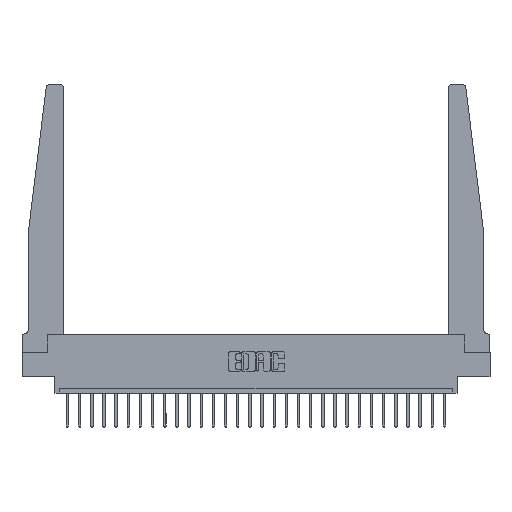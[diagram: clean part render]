
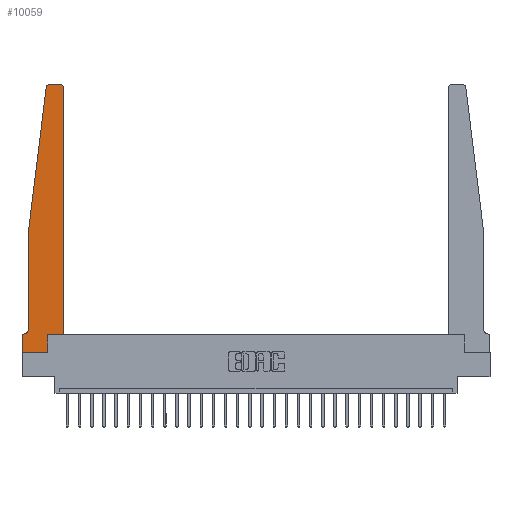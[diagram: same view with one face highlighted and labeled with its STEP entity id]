
A CAD part, top view. The second image highlights one B-rep face of the part: STEP entity #10059.
In plain terms, the highlighted planar face has unit normal (0, 0, 1).
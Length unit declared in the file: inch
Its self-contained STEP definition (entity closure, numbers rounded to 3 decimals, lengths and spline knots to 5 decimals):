
#682 = LINE ( 'NONE', #19217, #24742 ) ;
#1651 = DIRECTION ( 'NONE',  ( 0., 0., 1. ) ) ;
#1789 = DIRECTION ( 'NONE',  ( 1., 0., 0. ) ) ;
#1814 = LINE ( 'NONE', #2069, #9241 ) ;
#2069 = CARTESIAN_POINT ( 'NONE',  ( 0.065, 1.25, 0.37 ) ) ;
#2186 = ORIENTED_EDGE ( 'NONE', *, *, #5775, .T. ) ;
#2932 = VERTEX_POINT ( 'NONE', #6371 ) ;
#2943 = ORIENTED_EDGE ( 'NONE', *, *, #3992, .T. ) ;
#3528 = ORIENTED_EDGE ( 'NONE', *, *, #22419, .T. ) ;
#3712 = DIRECTION ( 'NONE',  ( 0., 0., 1. ) ) ;
#3728 = LINE ( 'NONE', #24303, #25688 ) ;
#3889 = DIRECTION ( 'NONE',  ( 0., 0., 1. ) ) ;
#3896 = CARTESIAN_POINT ( 'NONE',  ( 0., 0.1875, 0.37 ) ) ;
#3992 = EDGE_CURVE ( 'NONE', #25534, #2932, #1814, .T. ) ;
#4016 = ORIENTED_EDGE ( 'NONE', *, *, #21469, .T. ) ;
#4649 = CARTESIAN_POINT ( 'NONE',  ( 0.24675, 2.72367, 0.37 ) ) ;
#4956 = LINE ( 'NONE', #25655, #26504 ) ;
#5046 = AXIS2_PLACEMENT_3D ( 'NONE', #5643, #3889, #5364 ) ;
#5364 = DIRECTION ( 'NONE',  ( 1., 0., 0. ) ) ;
#5643 = CARTESIAN_POINT ( 'NONE',  ( 0.27653, 2.72, 0.37 ) ) ;
#5775 = EDGE_CURVE ( 'NONE', #13476, #9984, #17082, .T. ) ;
#5813 = ORIENTED_EDGE ( 'NONE', *, *, #13775, .T. ) ;
#6371 = CARTESIAN_POINT ( 'NONE',  ( 0.065, 1.25, 0.37 ) ) ;
#6737 = ORIENTED_EDGE ( 'NONE', *, *, #11946, .T. ) ;
#6999 = DIRECTION ( 'NONE',  ( 0., 1., 0. ) ) ;
#7258 = LINE ( 'NONE', #7387, #21319 ) ;
#7329 = CARTESIAN_POINT ( 'NONE',  ( 0.395, 2.75, 0.37 ) ) ;
#7387 = CARTESIAN_POINT ( 'NONE',  ( 0., 0., 0.37 ) ) ;
#7776 = VERTEX_POINT ( 'NONE', #12503 ) ;
#8574 = ORIENTED_EDGE ( 'NONE', *, *, #17228, .T. ) ;
#9241 = VECTOR ( 'NONE', #18085, 39.37008 ) ;
#9984 = VERTEX_POINT ( 'NONE', #13366 ) ;
#10033 = DIRECTION ( 'NONE',  ( 1., 0., 0. ) ) ;
#10059 = ADVANCED_FACE ( 'NONE', ( #26112 ), #22387, .T. ) ;
#10229 = VECTOR ( 'NONE', #24335, 39.37008 ) ;
#10693 = CARTESIAN_POINT ( 'NONE',  ( 0.27653, 2.75, 0.37 ) ) ;
#10754 = VERTEX_POINT ( 'NONE', #24577 ) ;
#10897 = DIRECTION ( 'NONE',  ( 1., 0., 0. ) ) ;
#11139 = DIRECTION ( 'NONE',  ( 0., -1., 0. ) ) ;
#11283 = DIRECTION ( 'NONE',  ( 1., 0., 0. ) ) ;
#11946 = EDGE_CURVE ( 'NONE', #23131, #25534, #17490, .T. ) ;
#12339 = ORIENTED_EDGE ( 'NONE', *, *, #20055, .T. ) ;
#12503 = CARTESIAN_POINT ( 'NONE',  ( 0.2605, 0.18, 0.37 ) ) ;
#12596 = DIRECTION ( 'NONE',  ( -1., 0., 0. ) ) ;
#13287 = LINE ( 'NONE', #17044, #17440 ) ;
#13366 = CARTESIAN_POINT ( 'NONE',  ( 0.015, 0.1875, 0.37 ) ) ;
#13476 = VERTEX_POINT ( 'NONE', #19071 ) ;
#13775 = EDGE_CURVE ( 'NONE', #9984, #14555, #16897, .T. ) ;
#14555 = VERTEX_POINT ( 'NONE', #3896 ) ;
#15235 = CARTESIAN_POINT ( 'NONE',  ( 0.425, 0.18, 0.37 ) ) ;
#15365 = CARTESIAN_POINT ( 'NONE',  ( 0.2605, 0., 0.37 ) ) ;
#16143 = ORIENTED_EDGE ( 'NONE', *, *, #19221, .T. ) ;
#16174 = DIRECTION ( 'NONE',  ( -1., 0., 0. ) ) ;
#16282 = LINE ( 'NONE', #24204, #10229 ) ;
#16313 = CARTESIAN_POINT ( 'NONE',  ( 0.015, 0.2375, 0.37 ) ) ;
#16369 = VERTEX_POINT ( 'NONE', #22849 ) ;
#16447 = DIRECTION ( 'NONE',  ( 0., 0., -1. ) ) ;
#16897 = LINE ( 'NONE', #20680, #26113 ) ;
#17044 = CARTESIAN_POINT ( 'NONE',  ( 0.065, 1.25, 0.37 ) ) ;
#17082 = CIRCLE ( 'NONE', #23110, 0.05 ) ;
#17181 = ORIENTED_EDGE ( 'NONE', *, *, #17191, .T. ) ;
#17191 = EDGE_CURVE ( 'NONE', #16369, #25927, #7258, .T. ) ;
#17228 = EDGE_CURVE ( 'NONE', #25927, #7776, #682, .T. ) ;
#17268 = AXIS2_PLACEMENT_3D ( 'NONE', #20354, #1651, #1789 ) ;
#17440 = VECTOR ( 'NONE', #11139, 39.37008 ) ;
#17490 = CIRCLE ( 'NONE', #5046, 0.03 ) ;
#18085 = DIRECTION ( 'NONE',  ( -0.122, -0.992, 0. ) ) ;
#18765 = VERTEX_POINT ( 'NONE', #20734 ) ;
#19071 = CARTESIAN_POINT ( 'NONE',  ( 0.065, 0.2375, 0.37 ) ) ;
#19217 = CARTESIAN_POINT ( 'NONE',  ( 0.2605, 0.18, 0.37 ) ) ;
#19221 = EDGE_CURVE ( 'NONE', #10754, #18765, #25847, .T. ) ;
#19421 = ORIENTED_EDGE ( 'NONE', *, *, #23416, .T. ) ;
#19594 = CIRCLE ( 'NONE', #19659, 0.03 ) ;
#19659 = AXIS2_PLACEMENT_3D ( 'NONE', #19866, #3712, #10033 ) ;
#19866 = CARTESIAN_POINT ( 'NONE',  ( 0.395, 2.72, 0.37 ) ) ;
#20055 = EDGE_CURVE ( 'NONE', #2932, #13476, #13287, .T. ) ;
#20354 = CARTESIAN_POINT ( 'NONE',  ( 0., 0.1875, 0.37 ) ) ;
#20680 = CARTESIAN_POINT ( 'NONE',  ( 0.065, 0.1875, 0.37 ) ) ;
#20734 = CARTESIAN_POINT ( 'NONE',  ( 0.425, 2.72, 0.37 ) ) ;
#20857 = ORIENTED_EDGE ( 'NONE', *, *, #23852, .T. ) ;
#21319 = VECTOR ( 'NONE', #10897, 39.37008 ) ;
#21469 = EDGE_CURVE ( 'NONE', #18765, #25606, #19594, .T. ) ;
#22387 = PLANE ( 'NONE',  #17268 ) ;
#22419 = EDGE_CURVE ( 'NONE', #7776, #10754, #4956, .T. ) ;
#22849 = CARTESIAN_POINT ( 'NONE',  ( 0., 0., 0.37 ) ) ;
#23110 = AXIS2_PLACEMENT_3D ( 'NONE', #16313, #16447, #16174 ) ;
#23131 = VERTEX_POINT ( 'NONE', #10693 ) ;
#23396 = EDGE_LOOP ( 'NONE', ( #19421, #6737, #2943, #12339, #2186, #5813, #20857, #17181, #8574, #3528, #16143, #4016 ) ) ;
#23416 = EDGE_CURVE ( 'NONE', #25606, #23131, #16282, .T. ) ;
#23852 = EDGE_CURVE ( 'NONE', #14555, #16369, #3728, .T. ) ;
#24053 = DIRECTION ( 'NONE',  ( 0., -1., 0. ) ) ;
#24204 = CARTESIAN_POINT ( 'NONE',  ( 0.25, 2.75, 0.37 ) ) ;
#24303 = CARTESIAN_POINT ( 'NONE',  ( 0., 0., 0.37 ) ) ;
#24335 = DIRECTION ( 'NONE',  ( -1., 0., 0. ) ) ;
#24577 = CARTESIAN_POINT ( 'NONE',  ( 0.425, 0.18, 0.37 ) ) ;
#24742 = VECTOR ( 'NONE', #6999, 39.37008 ) ;
#25325 = DIRECTION ( 'NONE',  ( 0., 1., 0. ) ) ;
#25534 = VERTEX_POINT ( 'NONE', #4649 ) ;
#25606 = VERTEX_POINT ( 'NONE', #7329 ) ;
#25655 = CARTESIAN_POINT ( 'NONE',  ( 0.425, 0.18, 0.37 ) ) ;
#25688 = VECTOR ( 'NONE', #24053, 39.37008 ) ;
#25847 = LINE ( 'NONE', #15235, #26443 ) ;
#25927 = VERTEX_POINT ( 'NONE', #15365 ) ;
#26112 = FACE_OUTER_BOUND ( 'NONE', #23396, .T. ) ;
#26113 = VECTOR ( 'NONE', #12596, 39.37008 ) ;
#26443 = VECTOR ( 'NONE', #25325, 39.37008 ) ;
#26504 = VECTOR ( 'NONE', #11283, 39.37008 ) ;
